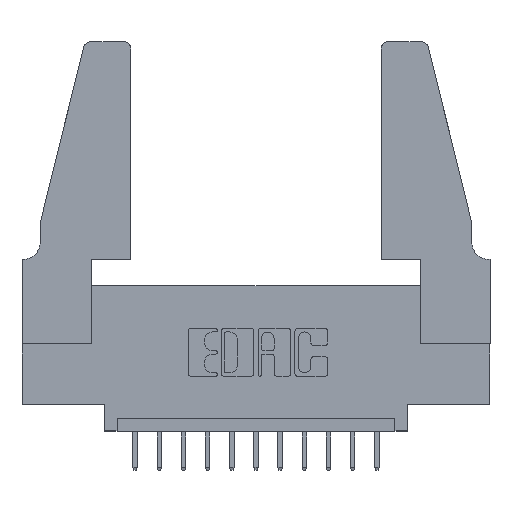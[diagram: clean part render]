
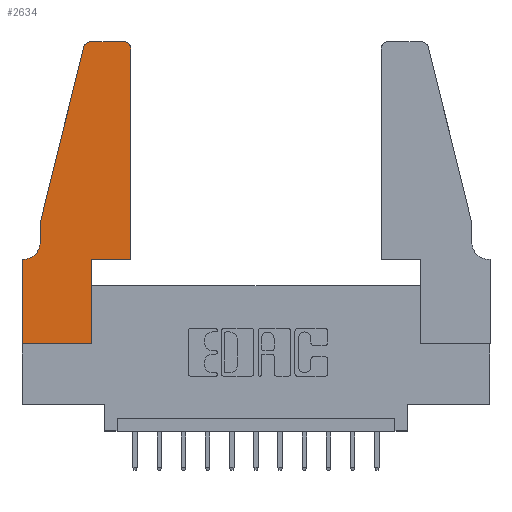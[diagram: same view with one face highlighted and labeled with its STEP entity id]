
A CAD part, top view. The second image highlights one B-rep face of the part: STEP entity #2634.
In plain terms, the highlighted planar face has unit normal (0, 0, 1).
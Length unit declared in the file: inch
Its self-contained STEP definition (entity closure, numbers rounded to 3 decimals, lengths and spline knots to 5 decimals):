
#154 = CARTESIAN_POINT ( 'NONE',  ( 0.2865, 0.35, 0.37 ) ) ;
#291 = LINE ( 'NONE', #3407, #12475 ) ;
#494 = CARTESIAN_POINT ( 'NONE',  ( 0.4505, 0.35, 0.37 ) ) ;
#700 = LINE ( 'NONE', #14319, #10395 ) ;
#898 = DIRECTION ( 'NONE',  ( -1., 0., 0. ) ) ;
#1188 = VERTEX_POINT ( 'NONE', #12732 ) ;
#1455 = CARTESIAN_POINT ( 'NONE',  ( 0.0055, 0.42, 0.37 ) ) ;
#1535 = LINE ( 'NONE', #14210, #2981 ) ;
#1709 = VERTEX_POINT ( 'NONE', #154 ) ;
#1783 = VERTEX_POINT ( 'NONE', #494 ) ;
#1945 = ORIENTED_EDGE ( 'NONE', *, *, #3810, .T. ) ;
#2171 = LINE ( 'NONE', #9153, #5379 ) ;
#2243 = VERTEX_POINT ( 'NONE', #2410 ) ;
#2410 = CARTESIAN_POINT ( 'NONE',  ( 0.0055, 0.35, 0.37 ) ) ;
#2499 = EDGE_CURVE ( 'NONE', #9543, #2243, #9670, .T. ) ;
#2634 = ADVANCED_FACE ( 'NONE', ( #5393 ), #9685, .T. ) ;
#2696 = ORIENTED_EDGE ( 'NONE', *, *, #6591, .T. ) ;
#2863 = LINE ( 'NONE', #5397, #8927 ) ;
#2981 = VECTOR ( 'NONE', #8810, 39.37008 ) ;
#2985 = EDGE_CURVE ( 'NONE', #14471, #1709, #9844, .T. ) ;
#3154 = LINE ( 'NONE', #7664, #12596 ) ;
#3290 = CARTESIAN_POINT ( 'NONE',  ( 0.4505, 0.35, 0.37 ) ) ;
#3301 = VERTEX_POINT ( 'NONE', #3648 ) ;
#3342 = DIRECTION ( 'NONE',  ( 0., -1., 0. ) ) ;
#3344 = DIRECTION ( 'NONE',  ( 0., 1., 0. ) ) ;
#3357 = DIRECTION ( 'NONE',  ( 0., 1., 0. ) ) ;
#3407 = CARTESIAN_POINT ( 'NONE',  ( 0.4505, 0.35, 0.37 ) ) ;
#3453 = CARTESIAN_POINT ( 'NONE',  ( 0.2865, 0.35, 0.37 ) ) ;
#3648 = CARTESIAN_POINT ( 'NONE',  ( 0.25487, 1.22718, 0.37 ) ) ;
#3651 = CARTESIAN_POINT ( 'NONE',  ( 0.284, 1.22, 0.37 ) ) ;
#3810 = EDGE_CURVE ( 'NONE', #11783, #13141, #14472, .T. ) ;
#3960 = DIRECTION ( 'NONE',  ( 1., 0., 0. ) ) ;
#3981 = CARTESIAN_POINT ( 'NONE',  ( 0.0755, 0.42, 0.37 ) ) ;
#4149 = VECTOR ( 'NONE', #3357, 39.37008 ) ;
#4197 = AXIS2_PLACEMENT_3D ( 'NONE', #1455, #12789, #7084 ) ;
#4730 = ORIENTED_EDGE ( 'NONE', *, *, #2499, .T. ) ;
#4782 = DIRECTION ( 'NONE',  ( 0., 0., 1. ) ) ;
#4949 = DIRECTION ( 'NONE',  ( 0., 0., 1. ) ) ;
#5112 = ORIENTED_EDGE ( 'NONE', *, *, #8195, .T. ) ;
#5379 = VECTOR ( 'NONE', #6705, 39.37008 ) ;
#5393 = FACE_OUTER_BOUND ( 'NONE', #10699, .T. ) ;
#5397 = CARTESIAN_POINT ( 'NONE',  ( 0.0755, 0.35, 0.37 ) ) ;
#5620 = AXIS2_PLACEMENT_3D ( 'NONE', #14161, #4949, #7290 ) ;
#5722 = VERTEX_POINT ( 'NONE', #14158 ) ;
#5783 = AXIS2_PLACEMENT_3D ( 'NONE', #3651, #4782, #8402 ) ;
#6102 = AXIS2_PLACEMENT_3D ( 'NONE', #7285, #6188, #12994 ) ;
#6188 = DIRECTION ( 'NONE',  ( 0., 0., 1. ) ) ;
#6591 = EDGE_CURVE ( 'NONE', #1783, #11783, #291, .T. ) ;
#6705 = DIRECTION ( 'NONE',  ( 0., -1., 0. ) ) ;
#7084 = DIRECTION ( 'NONE',  ( -1., 0., 0. ) ) ;
#7129 = ORIENTED_EDGE ( 'NONE', *, *, #13408, .T. ) ;
#7170 = CARTESIAN_POINT ( 'NONE',  ( 0.2865, 0., 0.37 ) ) ;
#7285 = CARTESIAN_POINT ( 'NONE',  ( 0.4205, 1.22, 0.37 ) ) ;
#7290 = DIRECTION ( 'NONE',  ( 1., 0., 0. ) ) ;
#7351 = EDGE_CURVE ( 'NONE', #1188, #9543, #9402, .T. ) ;
#7439 = ORIENTED_EDGE ( 'NONE', *, *, #7351, .T. ) ;
#7455 = CARTESIAN_POINT ( 'NONE',  ( 0., 0.35, 0.37 ) ) ;
#7664 = CARTESIAN_POINT ( 'NONE',  ( 0., 0., 0.37 ) ) ;
#8195 = EDGE_CURVE ( 'NONE', #13141, #5722, #1535, .T. ) ;
#8215 = EDGE_CURVE ( 'NONE', #9189, #14471, #3154, .T. ) ;
#8295 = ORIENTED_EDGE ( 'NONE', *, *, #2985, .T. ) ;
#8402 = DIRECTION ( 'NONE',  ( 1., 0., 0. ) ) ;
#8810 = DIRECTION ( 'NONE',  ( -1., 0., 0. ) ) ;
#8927 = VECTOR ( 'NONE', #898, 39.37008 ) ;
#9153 = CARTESIAN_POINT ( 'NONE',  ( 0., 0., 0.37 ) ) ;
#9189 = VERTEX_POINT ( 'NONE', #11575 ) ;
#9402 = LINE ( 'NONE', #12320, #9948 ) ;
#9499 = ORIENTED_EDGE ( 'NONE', *, *, #9549, .T. ) ;
#9543 = VERTEX_POINT ( 'NONE', #3981 ) ;
#9549 = EDGE_CURVE ( 'NONE', #1709, #1783, #14534, .T. ) ;
#9636 = CIRCLE ( 'NONE', #5783, 0.03 ) ;
#9670 = CIRCLE ( 'NONE', #4197, 0.07 ) ;
#9685 = PLANE ( 'NONE',  #5620 ) ;
#9844 = LINE ( 'NONE', #3453, #4149 ) ;
#9948 = VECTOR ( 'NONE', #3342, 39.37008 ) ;
#10395 = VECTOR ( 'NONE', #10595, 39.37008 ) ;
#10595 = DIRECTION ( 'NONE',  ( -0.239, -0.971, 0. ) ) ;
#10699 = EDGE_LOOP ( 'NONE', ( #5112, #13839, #14737, #7439, #4730, #7129, #11473, #13998, #8295, #9499, #2696, #1945 ) ) ;
#10772 = VERTEX_POINT ( 'NONE', #7455 ) ;
#11211 = EDGE_CURVE ( 'NONE', #3301, #1188, #700, .T. ) ;
#11473 = ORIENTED_EDGE ( 'NONE', *, *, #12430, .T. ) ;
#11575 = CARTESIAN_POINT ( 'NONE',  ( 0., 0., 0.37 ) ) ;
#11599 = EDGE_CURVE ( 'NONE', #5722, #3301, #9636, .T. ) ;
#11783 = VERTEX_POINT ( 'NONE', #13814 ) ;
#12320 = CARTESIAN_POINT ( 'NONE',  ( 0.0755, 0.5, 0.37 ) ) ;
#12430 = EDGE_CURVE ( 'NONE', #10772, #9189, #2171, .T. ) ;
#12475 = VECTOR ( 'NONE', #3344, 39.37008 ) ;
#12596 = VECTOR ( 'NONE', #12882, 39.37008 ) ;
#12732 = CARTESIAN_POINT ( 'NONE',  ( 0.0755, 0.5, 0.37 ) ) ;
#12789 = DIRECTION ( 'NONE',  ( 0., 0., -1. ) ) ;
#12882 = DIRECTION ( 'NONE',  ( 1., 0., 0. ) ) ;
#12930 = VECTOR ( 'NONE', #3960, 39.37008 ) ;
#12994 = DIRECTION ( 'NONE',  ( 1., 0., 0. ) ) ;
#13013 = CARTESIAN_POINT ( 'NONE',  ( 0.4205, 1.25, 0.37 ) ) ;
#13141 = VERTEX_POINT ( 'NONE', #13013 ) ;
#13408 = EDGE_CURVE ( 'NONE', #2243, #10772, #2863, .T. ) ;
#13814 = CARTESIAN_POINT ( 'NONE',  ( 0.4505, 1.22, 0.37 ) ) ;
#13839 = ORIENTED_EDGE ( 'NONE', *, *, #11599, .T. ) ;
#13998 = ORIENTED_EDGE ( 'NONE', *, *, #8215, .T. ) ;
#14158 = CARTESIAN_POINT ( 'NONE',  ( 0.284, 1.25, 0.37 ) ) ;
#14161 = CARTESIAN_POINT ( 'NONE',  ( 0., 0.35, 0.37 ) ) ;
#14210 = CARTESIAN_POINT ( 'NONE',  ( 0.2605, 1.25, 0.37 ) ) ;
#14319 = CARTESIAN_POINT ( 'NONE',  ( 0.0755, 0.5, 0.37 ) ) ;
#14471 = VERTEX_POINT ( 'NONE', #7170 ) ;
#14472 = CIRCLE ( 'NONE', #6102, 0.03 ) ;
#14534 = LINE ( 'NONE', #3290, #12930 ) ;
#14737 = ORIENTED_EDGE ( 'NONE', *, *, #11211, .T. ) ;
